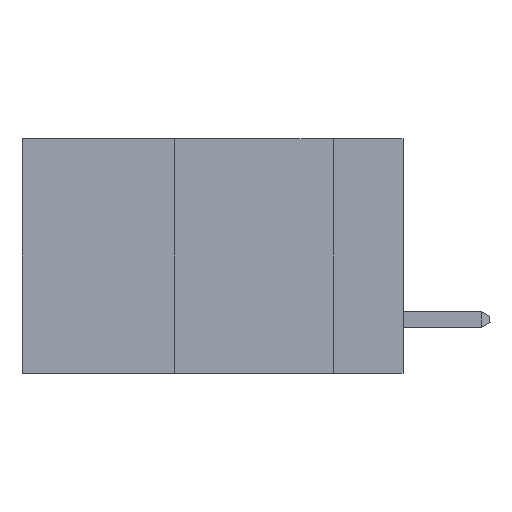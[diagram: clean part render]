
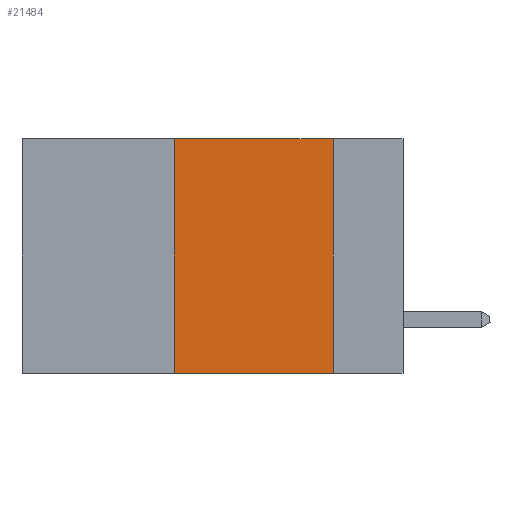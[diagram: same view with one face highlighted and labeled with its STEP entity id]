
A CAD part, left-side view. The second image highlights one B-rep face of the part: STEP entity #21484.
In plain terms, the highlighted planar face has unit normal (-1, 0, 0).
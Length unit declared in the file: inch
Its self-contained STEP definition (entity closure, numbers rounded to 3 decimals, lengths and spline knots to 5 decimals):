
#90 = DIRECTION ( 'NONE',  ( 0., -1., 0. ) ) ;
#647 = DIRECTION ( 'NONE',  ( 0., 0., -1. ) ) ;
#864 = VERTEX_POINT ( 'NONE', #10103 ) ;
#1041 = ORIENTED_EDGE ( 'NONE', *, *, #18780, .T. ) ;
#1654 = VERTEX_POINT ( 'NONE', #18521 ) ;
#2282 = EDGE_CURVE ( 'NONE', #20855, #1654, #11785, .T. ) ;
#4042 = AXIS2_PLACEMENT_3D ( 'NONE', #15738, #4263, #647 ) ;
#4263 = DIRECTION ( 'NONE',  ( 1., 0., 0. ) ) ;
#4599 = DIRECTION ( 'NONE',  ( 0., -1., 0. ) ) ;
#4785 = ORIENTED_EDGE ( 'NONE', *, *, #5308, .F. ) ;
#5308 = EDGE_CURVE ( 'NONE', #864, #20855, #23669, .T. ) ;
#5965 = ORIENTED_EDGE ( 'NONE', *, *, #12849, .F. ) ;
#7202 = VECTOR ( 'NONE', #23076, 39.37008 ) ;
#7231 = CARTESIAN_POINT ( 'NONE',  ( 0., 0.6, 0. ) ) ;
#7236 = CARTESIAN_POINT ( 'NONE',  ( 0., 0.36, -0.37 ) ) ;
#7689 = LINE ( 'NONE', #15769, #24088 ) ;
#9384 = DIRECTION ( 'NONE',  ( 0., 0., -1. ) ) ;
#10103 = CARTESIAN_POINT ( 'NONE',  ( 0., 0.36, 0. ) ) ;
#10344 = CARTESIAN_POINT ( 'NONE',  ( 0., 0.11, 0. ) ) ;
#11785 = LINE ( 'NONE', #22830, #23825 ) ;
#12849 = EDGE_CURVE ( 'NONE', #19107, #864, #22993, .T. ) ;
#14336 = VECTOR ( 'NONE', #90, 39.37008 ) ;
#14844 = EDGE_LOOP ( 'NONE', ( #22845, #4785, #5965, #1041 ) ) ;
#15738 = CARTESIAN_POINT ( 'NONE',  ( 0., 0.6, 0. ) ) ;
#15769 = CARTESIAN_POINT ( 'NONE',  ( 0., 0.6, -0.37 ) ) ;
#17585 = CARTESIAN_POINT ( 'NONE',  ( 0., 0.36, 0. ) ) ;
#18521 = CARTESIAN_POINT ( 'NONE',  ( 0., 0.11, -0.37 ) ) ;
#18780 = EDGE_CURVE ( 'NONE', #19107, #1654, #7689, .T. ) ;
#19107 = VERTEX_POINT ( 'NONE', #7236 ) ;
#20855 = VERTEX_POINT ( 'NONE', #10344 ) ;
#21151 = PLANE ( 'NONE',  #4042 ) ;
#21283 = FACE_OUTER_BOUND ( 'NONE', #14844, .T. ) ;
#21484 = ADVANCED_FACE ( 'NONE', ( #21283 ), #21151, .F. ) ;
#22830 = CARTESIAN_POINT ( 'NONE',  ( 0., 0.11, 0. ) ) ;
#22845 = ORIENTED_EDGE ( 'NONE', *, *, #2282, .F. ) ;
#22993 = LINE ( 'NONE', #17585, #7202 ) ;
#23076 = DIRECTION ( 'NONE',  ( 0., 0., 1. ) ) ;
#23669 = LINE ( 'NONE', #7231, #14336 ) ;
#23825 = VECTOR ( 'NONE', #9384, 39.37008 ) ;
#24088 = VECTOR ( 'NONE', #4599, 39.37008 ) ;
